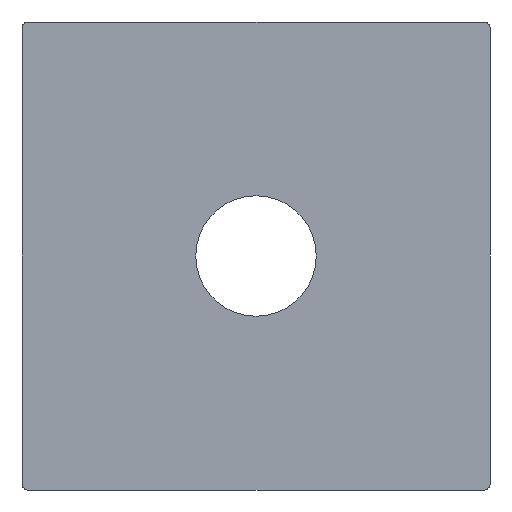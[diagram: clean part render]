
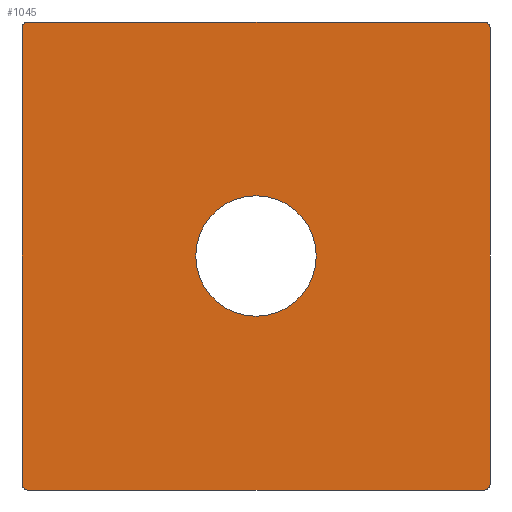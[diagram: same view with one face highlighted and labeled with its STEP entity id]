
A CAD part, front view. The second image highlights one B-rep face of the part: STEP entity #1045.
In plain terms, the highlighted planar face has unit normal (0, -1, 0).
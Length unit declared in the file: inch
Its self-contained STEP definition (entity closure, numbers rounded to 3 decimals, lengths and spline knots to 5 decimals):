
#113=LINE('',#1725,#198);
#114=LINE('',#1727,#199);
#151=LINE('',#1951,#236);
#152=LINE('',#1953,#237);
#198=VECTOR('',#1276,0.3937);
#199=VECTOR('',#1279,0.3937);
#236=VECTOR('',#1402,0.3937);
#237=VECTOR('',#1405,0.3937);
#259=PLANE('',#1150);
#264=FACE_BOUND('',#393,.T.);
#326=FACE_OUTER_BOUND('',#392,.T.);
#392=EDGE_LOOP('',(#954,#955,#956,#957,#958,#959,#960,#961));
#393=EDGE_LOOP('',(#962));
#395=CIRCLE('',#1068,0.2575);
#399=CIRCLE('',#1081,0.025);
#403=CIRCLE('',#1087,0.025);
#407=CIRCLE('',#1093,0.025);
#411=CIRCLE('',#1100,0.025);
#425=VERTEX_POINT('',#1412);
#463=VERTEX_POINT('',#1668);
#464=VERTEX_POINT('',#1669);
#468=VERTEX_POINT('',#1681);
#469=VERTEX_POINT('',#1682);
#473=VERTEX_POINT('',#1694);
#474=VERTEX_POINT('',#1695);
#478=VERTEX_POINT('',#1710);
#479=VERTEX_POINT('',#1711);
#517=EDGE_CURVE('',#425,#425,#395,.T.);
#572=EDGE_CURVE('',#463,#464,#399,.T.);
#578=EDGE_CURVE('',#468,#469,#403,.T.);
#584=EDGE_CURVE('',#473,#474,#407,.T.);
#592=EDGE_CURVE('',#478,#479,#411,.T.);
#601=EDGE_CURVE('',#463,#474,#113,.T.);
#602=EDGE_CURVE('',#473,#479,#114,.T.);
#663=EDGE_CURVE('',#468,#464,#151,.T.);
#664=EDGE_CURVE('',#478,#469,#152,.T.);
#954=ORIENTED_EDGE('',*,*,#572,.F.);
#955=ORIENTED_EDGE('',*,*,#601,.T.);
#956=ORIENTED_EDGE('',*,*,#584,.F.);
#957=ORIENTED_EDGE('',*,*,#602,.T.);
#958=ORIENTED_EDGE('',*,*,#592,.F.);
#959=ORIENTED_EDGE('',*,*,#664,.T.);
#960=ORIENTED_EDGE('',*,*,#578,.F.);
#961=ORIENTED_EDGE('',*,*,#663,.T.);
#962=ORIENTED_EDGE('',*,*,#517,.T.);
#1045=ADVANCED_FACE('',(#326,#264),#259,.F.);
#1068=AXIS2_PLACEMENT_3D('',#1413,#1157,#1158);
#1081=AXIS2_PLACEMENT_3D('',#1670,#1212,#1213);
#1087=AXIS2_PLACEMENT_3D('',#1683,#1226,#1227);
#1093=AXIS2_PLACEMENT_3D('',#1696,#1240,#1241);
#1100=AXIS2_PLACEMENT_3D('',#1712,#1258,#1259);
#1150=AXIS2_PLACEMENT_3D('',#1954,#1406,#1407);
#1157=DIRECTION('center_axis',(0.,1.,0.));
#1158=DIRECTION('ref_axis',(-1.,0.,0.));
#1212=DIRECTION('center_axis',(0.,1.,0.));
#1213=DIRECTION('ref_axis',(-0.707,0.,-0.707));
#1226=DIRECTION('center_axis',(0.,1.,0.));
#1227=DIRECTION('ref_axis',(-0.707,0.,0.707));
#1240=DIRECTION('center_axis',(0.,1.,0.));
#1241=DIRECTION('ref_axis',(0.707,0.,-0.707));
#1258=DIRECTION('center_axis',(0.,1.,0.));
#1259=DIRECTION('ref_axis',(0.707,0.,0.707));
#1276=DIRECTION('',(1.,0.,0.));
#1279=DIRECTION('',(0.,0.,1.));
#1402=DIRECTION('',(0.,0.,-1.));
#1405=DIRECTION('',(-1.,0.,0.));
#1406=DIRECTION('center_axis',(0.,1.,0.));
#1407=DIRECTION('ref_axis',(0.,0.,1.));
#1412=CARTESIAN_POINT('',(-0.7425,0.,-1.));
#1413=CARTESIAN_POINT('Origin',(-1.,0.,-1.));
#1668=CARTESIAN_POINT('',(-1.975,0.,-2.));
#1669=CARTESIAN_POINT('',(-2.,0.,-1.975));
#1670=CARTESIAN_POINT('Origin',(-1.975,0.,-1.975));
#1681=CARTESIAN_POINT('',(-2.,0.,-0.025));
#1682=CARTESIAN_POINT('',(-1.975,0.,0.));
#1683=CARTESIAN_POINT('Origin',(-1.975,0.,-0.025));
#1694=CARTESIAN_POINT('',(0.,0.,-1.975));
#1695=CARTESIAN_POINT('',(-0.025,0.,-2.));
#1696=CARTESIAN_POINT('Origin',(-0.025,0.,-1.975));
#1710=CARTESIAN_POINT('',(-0.025,0.,0.));
#1711=CARTESIAN_POINT('',(0.,0.,-0.025));
#1712=CARTESIAN_POINT('Origin',(-0.025,0.,-0.025));
#1725=CARTESIAN_POINT('',(-2.,0.,-2.));
#1727=CARTESIAN_POINT('',(0.,0.,-2.));
#1951=CARTESIAN_POINT('',(-2.,0.,0.));
#1953=CARTESIAN_POINT('',(0.,0.,0.));
#1954=CARTESIAN_POINT('Origin',(-1.,0.,-1.));
